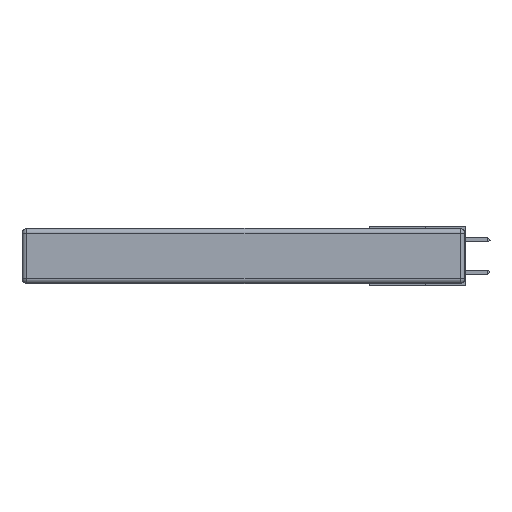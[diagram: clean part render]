
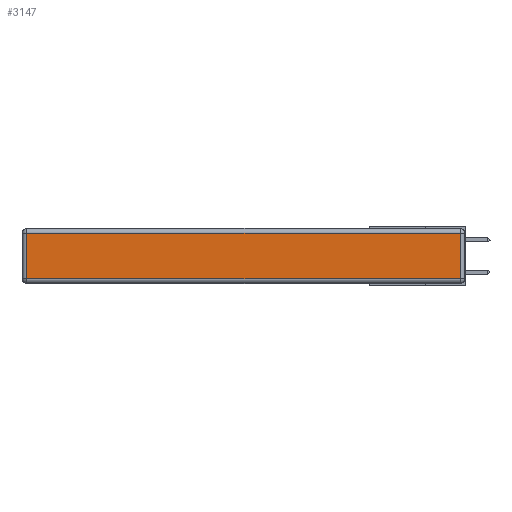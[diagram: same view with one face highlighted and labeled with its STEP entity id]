
A CAD part, left-side view. The second image highlights one B-rep face of the part: STEP entity #3147.
In plain terms, the highlighted planar face has unit normal (-1, 0, 0).
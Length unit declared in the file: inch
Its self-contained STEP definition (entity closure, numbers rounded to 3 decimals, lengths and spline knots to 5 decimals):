
#352 = DIRECTION ( 'NONE',  ( 0., 1., 0. ) ) ;
#426 = CARTESIAN_POINT ( 'NONE',  ( 0., 2.72, -0.313 ) ) ;
#1913 = LINE ( 'NONE', #15685, #10130 ) ;
#3046 = PLANE ( 'NONE',  #25208 ) ;
#3147 = ADVANCED_FACE ( 'NONE', ( #21293 ), #3046, .T. ) ;
#3715 = DIRECTION ( 'NONE',  ( -1., 0., 0. ) ) ;
#4897 = DIRECTION ( 'NONE',  ( 0., 0., -1. ) ) ;
#5459 = CARTESIAN_POINT ( 'NONE',  ( 0., 2.72, -0.03 ) ) ;
#5646 = VECTOR ( 'NONE', #10364, 39.37008 ) ;
#5908 = CARTESIAN_POINT ( 'NONE',  ( 0., 0., -0.313 ) ) ;
#7920 = CARTESIAN_POINT ( 'NONE',  ( 0., 0.03, -0.03 ) ) ;
#8551 = ORIENTED_EDGE ( 'NONE', *, *, #22208, .T. ) ;
#8649 = VERTEX_POINT ( 'NONE', #5459 ) ;
#9586 = ORIENTED_EDGE ( 'NONE', *, *, #22166, .T. ) ;
#10070 = VECTOR ( 'NONE', #14497, 39.37008 ) ;
#10130 = VECTOR ( 'NONE', #4897, 39.37008 ) ;
#10344 = VERTEX_POINT ( 'NONE', #426 ) ;
#10364 = DIRECTION ( 'NONE',  ( 0., -1., 0. ) ) ;
#10865 = EDGE_LOOP ( 'NONE', ( #9586, #8551, #11672, #24561 ) ) ;
#11672 = ORIENTED_EDGE ( 'NONE', *, *, #28156, .T. ) ;
#14497 = DIRECTION ( 'NONE',  ( 0., 0., 1. ) ) ;
#15280 = VERTEX_POINT ( 'NONE', #7920 ) ;
#15685 = CARTESIAN_POINT ( 'NONE',  ( 0., 2.72, -0.343 ) ) ;
#15696 = CARTESIAN_POINT ( 'NONE',  ( 0., 2.75, -0.03 ) ) ;
#16981 = CARTESIAN_POINT ( 'NONE',  ( 0., 0.03, -0.343 ) ) ;
#19990 = LINE ( 'NONE', #15696, #23769 ) ;
#20707 = EDGE_CURVE ( 'NONE', #8649, #10344, #1913, .T. ) ;
#21293 = FACE_OUTER_BOUND ( 'NONE', #10865, .T. ) ;
#22166 = EDGE_CURVE ( 'NONE', #10344, #25691, #22717, .T. ) ;
#22208 = EDGE_CURVE ( 'NONE', #25691, #15280, #26431, .T. ) ;
#22717 = LINE ( 'NONE', #5908, #5646 ) ;
#23477 = CARTESIAN_POINT ( 'NONE',  ( 0., 0.03, -0.313 ) ) ;
#23769 = VECTOR ( 'NONE', #352, 39.37008 ) ;
#24561 = ORIENTED_EDGE ( 'NONE', *, *, #20707, .T. ) ;
#24883 = CARTESIAN_POINT ( 'NONE',  ( 0., 0., -0.343 ) ) ;
#25208 = AXIS2_PLACEMENT_3D ( 'NONE', #24883, #3715, #27829 ) ;
#25691 = VERTEX_POINT ( 'NONE', #23477 ) ;
#26431 = LINE ( 'NONE', #16981, #10070 ) ;
#27829 = DIRECTION ( 'NONE',  ( 0., 0., 1. ) ) ;
#28156 = EDGE_CURVE ( 'NONE', #15280, #8649, #19990, .T. ) ;
